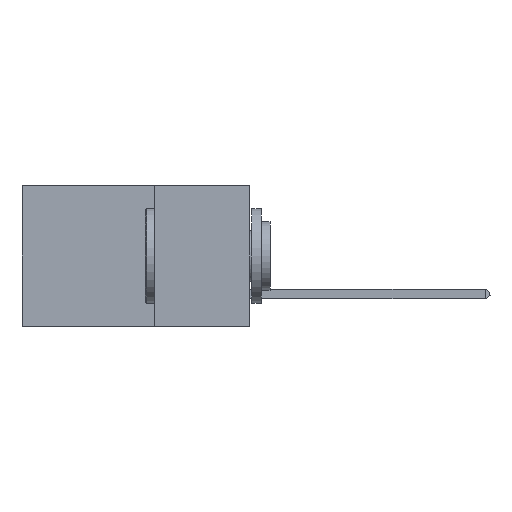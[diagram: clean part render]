
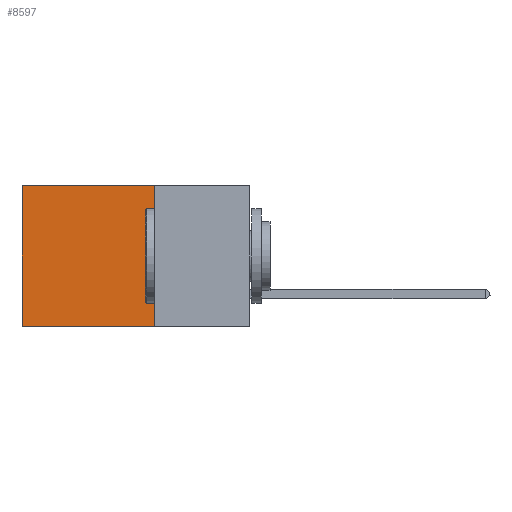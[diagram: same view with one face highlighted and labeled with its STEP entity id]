
A CAD part, left-side view. The second image highlights one B-rep face of the part: STEP entity #8597.
In plain terms, the highlighted planar face has unit normal (-1, 0, 0).
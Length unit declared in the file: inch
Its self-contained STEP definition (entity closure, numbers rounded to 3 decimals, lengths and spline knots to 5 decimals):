
#430 = CARTESIAN_POINT ( 'NONE',  ( 0.2875, 0.6, 0. ) ) ;
#2539 = CARTESIAN_POINT ( 'NONE',  ( 0.2875, 0.25, -0.37 ) ) ;
#6468 = VERTEX_POINT ( 'NONE', #22040 ) ;
#6699 = AXIS2_PLACEMENT_3D ( 'NONE', #41115, #16269, #44188 ) ;
#6993 = VECTOR ( 'NONE', #33671, 39.37008 ) ;
#8597 = ADVANCED_FACE ( 'NONE', ( #41325 ), #33865, .F. ) ;
#10326 = EDGE_CURVE ( 'NONE', #31037, #43566, #25820, .T. ) ;
#10353 = ORIENTED_EDGE ( 'NONE', *, *, #31446, .T. ) ;
#10479 = LINE ( 'NONE', #16890, #19816 ) ;
#10927 = CARTESIAN_POINT ( 'NONE',  ( 0.2875, 0.25, 0. ) ) ;
#11263 = DIRECTION ( 'NONE',  ( 0., 0., -1. ) ) ;
#13584 = EDGE_CURVE ( 'NONE', #6468, #38582, #24947, .T. ) ;
#15448 = ORIENTED_EDGE ( 'NONE', *, *, #10326, .F. ) ;
#15902 = CARTESIAN_POINT ( 'NONE',  ( 0.2875, 0.25, -0.37 ) ) ;
#16269 = DIRECTION ( 'NONE',  ( 1., 0., 0. ) ) ;
#16852 = EDGE_LOOP ( 'NONE', ( #38992, #16993, #15448, #10353 ) ) ;
#16890 = CARTESIAN_POINT ( 'NONE',  ( 0.2875, 0.25, 0. ) ) ;
#16993 = ORIENTED_EDGE ( 'NONE', *, *, #34338, .F. ) ;
#19816 = VECTOR ( 'NONE', #27600, 39.37008 ) ;
#22040 = CARTESIAN_POINT ( 'NONE',  ( 0.2875, 0.6, 0. ) ) ;
#24947 = LINE ( 'NONE', #430, #33200 ) ;
#25820 = LINE ( 'NONE', #10927, #42171 ) ;
#27600 = DIRECTION ( 'NONE',  ( 0., 1., 0. ) ) ;
#28545 = DIRECTION ( 'NONE',  ( 0., 0., -1. ) ) ;
#31037 = VERTEX_POINT ( 'NONE', #39330 ) ;
#31446 = EDGE_CURVE ( 'NONE', #31037, #6468, #10479, .T. ) ;
#33200 = VECTOR ( 'NONE', #11263, 39.37008 ) ;
#33671 = DIRECTION ( 'NONE',  ( 0., 1., 0. ) ) ;
#33865 = PLANE ( 'NONE',  #6699 ) ;
#34338 = EDGE_CURVE ( 'NONE', #43566, #38582, #38142, .T. ) ;
#36405 = CARTESIAN_POINT ( 'NONE',  ( 0.2875, 0.6, -0.37 ) ) ;
#38142 = LINE ( 'NONE', #15902, #6993 ) ;
#38582 = VERTEX_POINT ( 'NONE', #36405 ) ;
#38992 = ORIENTED_EDGE ( 'NONE', *, *, #13584, .T. ) ;
#39330 = CARTESIAN_POINT ( 'NONE',  ( 0.2875, 0.25, 0. ) ) ;
#41115 = CARTESIAN_POINT ( 'NONE',  ( 0.2875, 0.25, 0. ) ) ;
#41325 = FACE_OUTER_BOUND ( 'NONE', #16852, .T. ) ;
#42171 = VECTOR ( 'NONE', #28545, 39.37008 ) ;
#43566 = VERTEX_POINT ( 'NONE', #2539 ) ;
#44188 = DIRECTION ( 'NONE',  ( 0., 0., -1. ) ) ;
